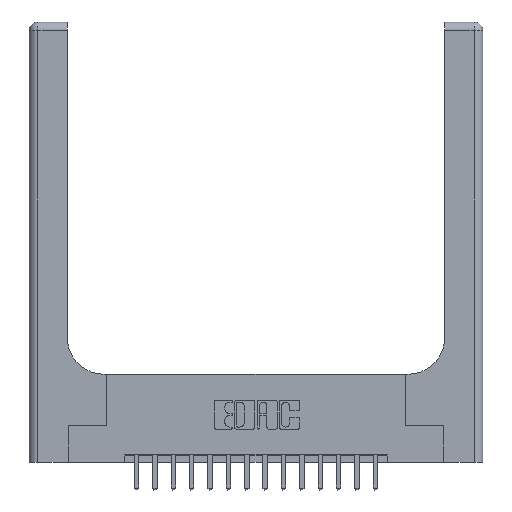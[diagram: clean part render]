
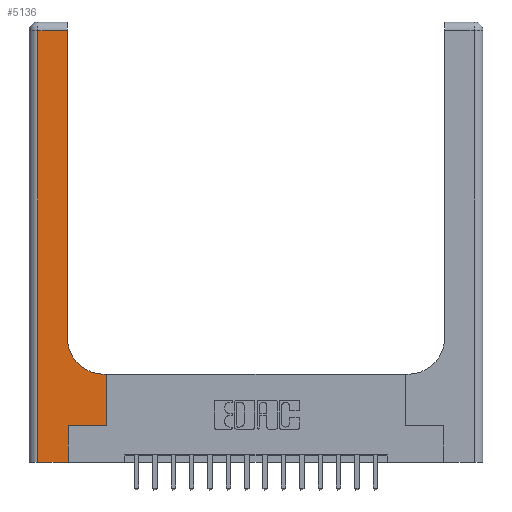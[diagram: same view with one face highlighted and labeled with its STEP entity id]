
A CAD part, top view. The second image highlights one B-rep face of the part: STEP entity #5136.
In plain terms, the highlighted planar face has unit normal (0, 0, 1).
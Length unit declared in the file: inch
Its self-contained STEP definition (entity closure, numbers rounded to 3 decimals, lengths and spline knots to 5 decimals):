
#90 = CARTESIAN_POINT ( 'NONE',  ( 0., 0., 0.37 ) ) ;
#110 = EDGE_CURVE ( 'NONE', #11792, #12242, #6446, .T. ) ;
#357 = EDGE_CURVE ( 'NONE', #5938, #13623, #10162, .T. ) ;
#455 = ORIENTED_EDGE ( 'NONE', *, *, #7176, .T. ) ;
#499 = ORIENTED_EDGE ( 'NONE', *, *, #357, .T. ) ;
#504 = ORIENTED_EDGE ( 'NONE', *, *, #1850, .T. ) ;
#959 = CARTESIAN_POINT ( 'NONE',  ( 0.528, 0.25, 0.37 ) ) ;
#1527 = DIRECTION ( 'NONE',  ( 0., 1., 0. ) ) ;
#1646 = CARTESIAN_POINT ( 'NONE',  ( 0.26, 2.94, 0.37 ) ) ;
#1748 = CARTESIAN_POINT ( 'NONE',  ( 0.26, 3., 0.37 ) ) ;
#1850 = EDGE_CURVE ( 'NONE', #13623, #11792, #17850, .T. ) ;
#1900 = DIRECTION ( 'NONE',  ( -1., 0., 0. ) ) ;
#2071 = VERTEX_POINT ( 'NONE', #16586 ) ;
#2645 = EDGE_LOOP ( 'NONE', ( #455, #8217, #499, #504, #9276, #5659, #11565, #6682, #8044 ) ) ;
#3115 = DIRECTION ( 'NONE',  ( 0., 0., -1. ) ) ;
#3577 = CARTESIAN_POINT ( 'NONE',  ( 0., 2.94, 0.37 ) ) ;
#3983 = EDGE_CURVE ( 'NONE', #2071, #16506, #6330, .T. ) ;
#4373 = EDGE_CURVE ( 'NONE', #8404, #2071, #17351, .T. ) ;
#4688 = VERTEX_POINT ( 'NONE', #5929 ) ;
#4889 = VECTOR ( 'NONE', #15292, 39.37008 ) ;
#5087 = EDGE_CURVE ( 'NONE', #12242, #4688, #12908, .T. ) ;
#5136 = ADVANCED_FACE ( 'NONE', ( #7155 ), #11424, .F. ) ;
#5155 = VECTOR ( 'NONE', #1527, 39.37008 ) ;
#5416 = VECTOR ( 'NONE', #13724, 39.37008 ) ;
#5659 = ORIENTED_EDGE ( 'NONE', *, *, #5087, .T. ) ;
#5752 = CARTESIAN_POINT ( 'NONE',  ( 0.26, 0.85, 0.37 ) ) ;
#5774 = AXIS2_PLACEMENT_3D ( 'NONE', #6754, #3115, #9995 ) ;
#5929 = CARTESIAN_POINT ( 'NONE',  ( 0.528, 0.25, 0.37 ) ) ;
#5938 = VERTEX_POINT ( 'NONE', #15459 ) ;
#6330 = CIRCLE ( 'NONE', #7139, 0.25 ) ;
#6446 = LINE ( 'NONE', #8503, #13513 ) ;
#6682 = ORIENTED_EDGE ( 'NONE', *, *, #4373, .T. ) ;
#6754 = CARTESIAN_POINT ( 'NONE',  ( 0., 3., 0.37 ) ) ;
#7139 = AXIS2_PLACEMENT_3D ( 'NONE', #8095, #13814, #9703 ) ;
#7155 = FACE_OUTER_BOUND ( 'NONE', #2645, .T. ) ;
#7176 = EDGE_CURVE ( 'NONE', #16506, #10253, #12651, .T. ) ;
#7440 = VECTOR ( 'NONE', #13681, 39.37008 ) ;
#8044 = ORIENTED_EDGE ( 'NONE', *, *, #3983, .T. ) ;
#8095 = CARTESIAN_POINT ( 'NONE',  ( 0.51, 0.85, 0.37 ) ) ;
#8217 = ORIENTED_EDGE ( 'NONE', *, *, #9071, .T. ) ;
#8404 = VERTEX_POINT ( 'NONE', #17899 ) ;
#8503 = CARTESIAN_POINT ( 'NONE',  ( 0.265, 0., 0.37 ) ) ;
#9071 = EDGE_CURVE ( 'NONE', #10253, #5938, #17863, .T. ) ;
#9276 = ORIENTED_EDGE ( 'NONE', *, *, #110, .T. ) ;
#9703 = DIRECTION ( 'NONE',  ( 1., 0., 0. ) ) ;
#9922 = CARTESIAN_POINT ( 'NONE',  ( 0.06, 3., 0.37 ) ) ;
#9995 = DIRECTION ( 'NONE',  ( -1., 0., 0. ) ) ;
#10162 = LINE ( 'NONE', #9922, #4889 ) ;
#10253 = VERTEX_POINT ( 'NONE', #1646 ) ;
#11148 = DIRECTION ( 'NONE',  ( 1., 0., 0. ) ) ;
#11213 = LINE ( 'NONE', #959, #7440 ) ;
#11424 = PLANE ( 'NONE',  #5774 ) ;
#11442 = VECTOR ( 'NONE', #11148, 39.37008 ) ;
#11565 = ORIENTED_EDGE ( 'NONE', *, *, #15197, .T. ) ;
#11685 = CARTESIAN_POINT ( 'NONE',  ( 0.265, 0., 0.37 ) ) ;
#11792 = VERTEX_POINT ( 'NONE', #11685 ) ;
#11820 = VECTOR ( 'NONE', #1900, 39.37008 ) ;
#12189 = CARTESIAN_POINT ( 'NONE',  ( 0.265, 0.25, 0.37 ) ) ;
#12242 = VERTEX_POINT ( 'NONE', #15770 ) ;
#12651 = LINE ( 'NONE', #1748, #5155 ) ;
#12908 = LINE ( 'NONE', #12189, #5416 ) ;
#13453 = DIRECTION ( 'NONE',  ( -1., 0., 0. ) ) ;
#13513 = VECTOR ( 'NONE', #17364, 39.37008 ) ;
#13623 = VERTEX_POINT ( 'NONE', #14557 ) ;
#13681 = DIRECTION ( 'NONE',  ( 0., 1., 0. ) ) ;
#13724 = DIRECTION ( 'NONE',  ( 1., 0., 0. ) ) ;
#13814 = DIRECTION ( 'NONE',  ( 0., 0., -1. ) ) ;
#14340 = VECTOR ( 'NONE', #13453, 39.37008 ) ;
#14557 = CARTESIAN_POINT ( 'NONE',  ( 0.06, 0., 0.37 ) ) ;
#14643 = CARTESIAN_POINT ( 'NONE',  ( 0.26, 0.6, 0.37 ) ) ;
#15197 = EDGE_CURVE ( 'NONE', #4688, #8404, #11213, .T. ) ;
#15292 = DIRECTION ( 'NONE',  ( 0., -1., 0. ) ) ;
#15459 = CARTESIAN_POINT ( 'NONE',  ( 0.06, 2.94, 0.37 ) ) ;
#15770 = CARTESIAN_POINT ( 'NONE',  ( 0.265, 0.25, 0.37 ) ) ;
#16506 = VERTEX_POINT ( 'NONE', #5752 ) ;
#16586 = CARTESIAN_POINT ( 'NONE',  ( 0.51, 0.6, 0.37 ) ) ;
#17351 = LINE ( 'NONE', #14643, #11820 ) ;
#17364 = DIRECTION ( 'NONE',  ( 0., 1., 0. ) ) ;
#17850 = LINE ( 'NONE', #90, #11442 ) ;
#17863 = LINE ( 'NONE', #3577, #14340 ) ;
#17899 = CARTESIAN_POINT ( 'NONE',  ( 0.528, 0.6, 0.37 ) ) ;
